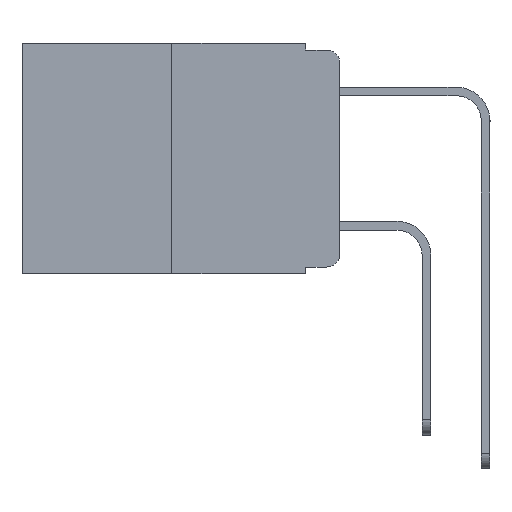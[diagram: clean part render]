
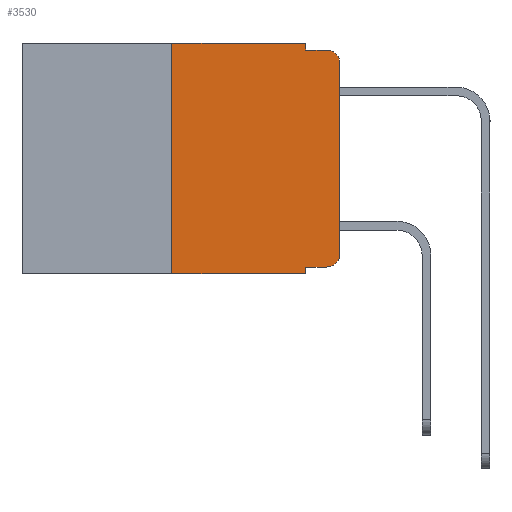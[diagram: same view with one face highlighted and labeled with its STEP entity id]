
A CAD part, left-side view. The second image highlights one B-rep face of the part: STEP entity #3530.
In plain terms, the highlighted planar face has unit normal (-1, 0, 0).
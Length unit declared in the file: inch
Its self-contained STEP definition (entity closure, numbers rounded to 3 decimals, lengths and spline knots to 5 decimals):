
#5 = PLANE ( 'NONE',  #1941 ) ;
#108 = CARTESIAN_POINT ( 'NONE',  ( 0., 0.051, 0. ) ) ;
#220 = DIRECTION ( 'NONE',  ( 0., 0., 1. ) ) ;
#1073 = VECTOR ( 'NONE', #21027, 39.37008 ) ;
#1275 = ORIENTED_EDGE ( 'NONE', *, *, #8213, .T. ) ;
#1291 = LINE ( 'NONE', #15532, #18799 ) ;
#1859 = VECTOR ( 'NONE', #17210, 39.37008 ) ;
#1872 = VERTEX_POINT ( 'NONE', #16806 ) ;
#1941 = AXIS2_PLACEMENT_3D ( 'NONE', #5156, #17039, #6893 ) ;
#2266 = CARTESIAN_POINT ( 'NONE',  ( 0., 0.051, 0. ) ) ;
#2381 = AXIS2_PLACEMENT_3D ( 'NONE', #5958, #17821, #7689 ) ;
#2390 = LINE ( 'NONE', #12158, #1859 ) ;
#2485 = VERTEX_POINT ( 'NONE', #108 ) ;
#2685 = VERTEX_POINT ( 'NONE', #14319 ) ;
#2857 = CARTESIAN_POINT ( 'NONE',  ( 0., 0.473, -0.343 ) ) ;
#3084 = ORIENTED_EDGE ( 'NONE', *, *, #10524, .F. ) ;
#3193 = VERTEX_POINT ( 'NONE', #5936 ) ;
#3530 = ADVANCED_FACE ( 'NONE', ( #17921 ), #5, .F. ) ;
#3885 = ORIENTED_EDGE ( 'NONE', *, *, #13959, .F. ) ;
#4551 = DIRECTION ( 'NONE',  ( 0., -1., 0. ) ) ;
#4631 = CARTESIAN_POINT ( 'NONE',  ( 0., 0.051, -0.01 ) ) ;
#4751 = EDGE_CURVE ( 'NONE', #18753, #5228, #14390, .T. ) ;
#4786 = CARTESIAN_POINT ( 'NONE',  ( 0., 0., -0.313 ) ) ;
#5156 = CARTESIAN_POINT ( 'NONE',  ( 0., 0.473, 0. ) ) ;
#5228 = VERTEX_POINT ( 'NONE', #4786 ) ;
#5564 = CARTESIAN_POINT ( 'NONE',  ( 0., 0.25, 0. ) ) ;
#5936 = CARTESIAN_POINT ( 'NONE',  ( 0., 0.02, -0.01 ) ) ;
#5958 = CARTESIAN_POINT ( 'NONE',  ( 0., 0.02, -0.03 ) ) ;
#6084 = VECTOR ( 'NONE', #4551, 39.37008 ) ;
#6326 = DIRECTION ( 'NONE',  ( 0., -1., 0. ) ) ;
#6565 = VECTOR ( 'NONE', #6326, 39.37008 ) ;
#6597 = CARTESIAN_POINT ( 'NONE',  ( 0., 0.051, -0.343 ) ) ;
#6697 = DIRECTION ( 'NONE',  ( -1., 0., 0. ) ) ;
#6893 = DIRECTION ( 'NONE',  ( 0., 0., -1. ) ) ;
#6945 = VECTOR ( 'NONE', #16188, 39.37008 ) ;
#7498 = LINE ( 'NONE', #21279, #6945 ) ;
#7583 = VECTOR ( 'NONE', #14880, 39.37008 ) ;
#7689 = DIRECTION ( 'NONE',  ( 0., 0., -1. ) ) ;
#7712 = LINE ( 'NONE', #4631, #6084 ) ;
#7782 = ORIENTED_EDGE ( 'NONE', *, *, #16190, .T. ) ;
#8105 = LINE ( 'NONE', #19874, #7583 ) ;
#8213 = EDGE_CURVE ( 'NONE', #21343, #18753, #8105, .T. ) ;
#8968 = CARTESIAN_POINT ( 'NONE',  ( 0., 0., -0.03 ) ) ;
#9370 = EDGE_CURVE ( 'NONE', #21343, #20023, #14726, .T. ) ;
#9903 = ORIENTED_EDGE ( 'NONE', *, *, #19512, .T. ) ;
#10070 = CARTESIAN_POINT ( 'NONE',  ( 0., 0.051, -0.333 ) ) ;
#10524 = EDGE_CURVE ( 'NONE', #1872, #11187, #1291, .T. ) ;
#11187 = VERTEX_POINT ( 'NONE', #5564 ) ;
#12158 = CARTESIAN_POINT ( 'NONE',  ( 0., 0., 0. ) ) ;
#12234 = ORIENTED_EDGE ( 'NONE', *, *, #17585, .T. ) ;
#12877 = EDGE_LOOP ( 'NONE', ( #9903, #7782, #19287, #3885, #13572, #3084, #12234, #21933, #1275, #15195 ) ) ;
#13572 = ORIENTED_EDGE ( 'NONE', *, *, #16346, .F. ) ;
#13959 = EDGE_CURVE ( 'NONE', #2485, #2685, #7498, .T. ) ;
#14319 = CARTESIAN_POINT ( 'NONE',  ( 0., 0.051, -0.01 ) ) ;
#14380 = VERTEX_POINT ( 'NONE', #8968 ) ;
#14390 = CIRCLE ( 'NONE', #15560, 0.02 ) ;
#14726 = LINE ( 'NONE', #2266, #1073 ) ;
#14880 = DIRECTION ( 'NONE',  ( 0., -1., 0. ) ) ;
#15080 = EDGE_CURVE ( 'NONE', #2685, #3193, #7712, .T. ) ;
#15195 = ORIENTED_EDGE ( 'NONE', *, *, #4751, .T. ) ;
#15337 = LINE ( 'NONE', #2857, #19207 ) ;
#15532 = CARTESIAN_POINT ( 'NONE',  ( 0., 0.25, 0. ) ) ;
#15560 = AXIS2_PLACEMENT_3D ( 'NONE', #16857, #6697, #18510 ) ;
#16188 = DIRECTION ( 'NONE',  ( 0., 0., -1. ) ) ;
#16190 = EDGE_CURVE ( 'NONE', #14380, #3193, #19259, .T. ) ;
#16346 = EDGE_CURVE ( 'NONE', #11187, #2485, #19507, .T. ) ;
#16503 = CARTESIAN_POINT ( 'NONE',  ( 0., 0.473, 0. ) ) ;
#16520 = DIRECTION ( 'NONE',  ( 0., -1., 0. ) ) ;
#16806 = CARTESIAN_POINT ( 'NONE',  ( 0., 0.25, -0.343 ) ) ;
#16857 = CARTESIAN_POINT ( 'NONE',  ( 0., 0.02, -0.313 ) ) ;
#17039 = DIRECTION ( 'NONE',  ( 1., 0., 0. ) ) ;
#17210 = DIRECTION ( 'NONE',  ( 0., 0., 1. ) ) ;
#17585 = EDGE_CURVE ( 'NONE', #1872, #20023, #15337, .T. ) ;
#17821 = DIRECTION ( 'NONE',  ( -1., 0., 0. ) ) ;
#17921 = FACE_OUTER_BOUND ( 'NONE', #12877, .T. ) ;
#18510 = DIRECTION ( 'NONE',  ( 0., 0., -1. ) ) ;
#18753 = VERTEX_POINT ( 'NONE', #20161 ) ;
#18799 = VECTOR ( 'NONE', #220, 39.37008 ) ;
#19207 = VECTOR ( 'NONE', #16520, 39.37008 ) ;
#19259 = CIRCLE ( 'NONE', #2381, 0.02 ) ;
#19287 = ORIENTED_EDGE ( 'NONE', *, *, #15080, .F. ) ;
#19507 = LINE ( 'NONE', #16503, #6565 ) ;
#19512 = EDGE_CURVE ( 'NONE', #5228, #14380, #2390, .T. ) ;
#19874 = CARTESIAN_POINT ( 'NONE',  ( 0., 0.051, -0.333 ) ) ;
#20023 = VERTEX_POINT ( 'NONE', #6597 ) ;
#20161 = CARTESIAN_POINT ( 'NONE',  ( 0., 0.02, -0.333 ) ) ;
#21027 = DIRECTION ( 'NONE',  ( 0., 0., -1. ) ) ;
#21279 = CARTESIAN_POINT ( 'NONE',  ( 0., 0.051, 0. ) ) ;
#21343 = VERTEX_POINT ( 'NONE', #10070 ) ;
#21933 = ORIENTED_EDGE ( 'NONE', *, *, #9370, .F. ) ;
